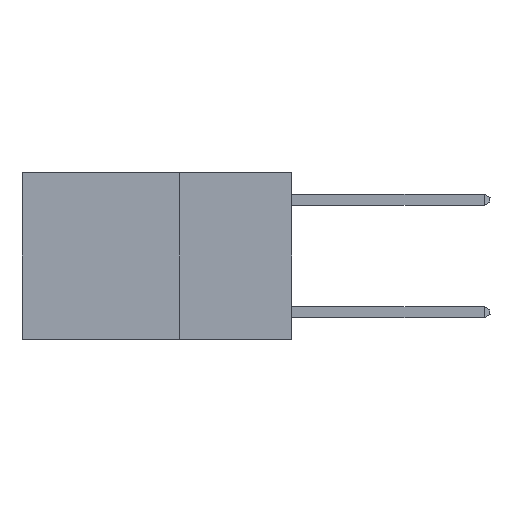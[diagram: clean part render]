
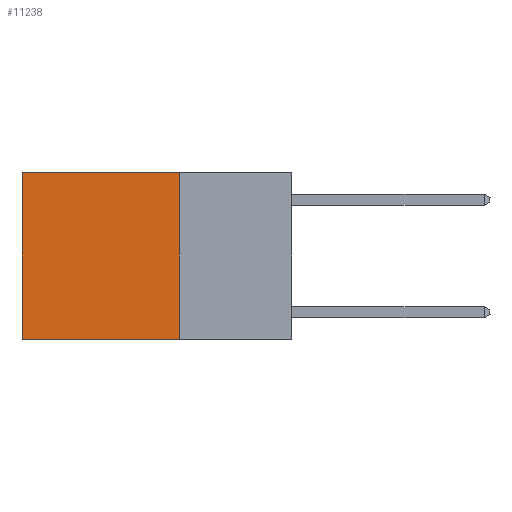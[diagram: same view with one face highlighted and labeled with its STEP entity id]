
A CAD part, left-side view. The second image highlights one B-rep face of the part: STEP entity #11238.
In plain terms, the highlighted planar face has unit normal (-1, 0, 0).
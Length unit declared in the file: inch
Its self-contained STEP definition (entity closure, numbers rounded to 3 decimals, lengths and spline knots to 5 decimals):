
#339 = DIRECTION ( 'NONE',  ( 1., 0., 0. ) ) ;
#448 = VERTEX_POINT ( 'NONE', #9764 ) ;
#543 = ORIENTED_EDGE ( 'NONE', *, *, #3418, .F. ) ;
#803 = CARTESIAN_POINT ( 'NONE',  ( 0.2625, 0.25, 0. ) ) ;
#977 = LINE ( 'NONE', #1709, #9962 ) ;
#1011 = EDGE_CURVE ( 'NONE', #10514, #448, #5418, .T. ) ;
#1025 = LINE ( 'NONE', #6963, #1721 ) ;
#1190 = PLANE ( 'NONE',  #1799 ) ;
#1346 = VECTOR ( 'NONE', #2040, 39.37008 ) ;
#1400 = EDGE_LOOP ( 'NONE', ( #9079, #543, #10496, #2004 ) ) ;
#1709 = CARTESIAN_POINT ( 'NONE',  ( 0.2625, 0.25, -0.37 ) ) ;
#1721 = VECTOR ( 'NONE', #9703, 39.37008 ) ;
#1765 = DIRECTION ( 'NONE',  ( 0., 1., 0. ) ) ;
#1799 = AXIS2_PLACEMENT_3D ( 'NONE', #9866, #339, #7353 ) ;
#1936 = LINE ( 'NONE', #3790, #5682 ) ;
#2004 = ORIENTED_EDGE ( 'NONE', *, *, #7524, .T. ) ;
#2040 = DIRECTION ( 'NONE',  ( 0., 0., -1. ) ) ;
#2879 = DIRECTION ( 'NONE',  ( 0., 1., 0. ) ) ;
#3418 = EDGE_CURVE ( 'NONE', #448, #3503, #977, .T. ) ;
#3503 = VERTEX_POINT ( 'NONE', #10348 ) ;
#3790 = CARTESIAN_POINT ( 'NONE',  ( 0.2625, 0.25, 0. ) ) ;
#3941 = CARTESIAN_POINT ( 'NONE',  ( 0.2625, 0.25, 0. ) ) ;
#5418 = LINE ( 'NONE', #3941, #1346 ) ;
#5682 = VECTOR ( 'NONE', #2879, 39.37008 ) ;
#6334 = VERTEX_POINT ( 'NONE', #6745 ) ;
#6586 = EDGE_CURVE ( 'NONE', #6334, #3503, #1025, .T. ) ;
#6745 = CARTESIAN_POINT ( 'NONE',  ( 0.2625, 0.6, 0. ) ) ;
#6963 = CARTESIAN_POINT ( 'NONE',  ( 0.2625, 0.6, 0. ) ) ;
#7353 = DIRECTION ( 'NONE',  ( 0., 0., -1. ) ) ;
#7524 = EDGE_CURVE ( 'NONE', #10514, #6334, #1936, .T. ) ;
#9008 = FACE_OUTER_BOUND ( 'NONE', #1400, .T. ) ;
#9079 = ORIENTED_EDGE ( 'NONE', *, *, #6586, .T. ) ;
#9703 = DIRECTION ( 'NONE',  ( 0., 0., -1. ) ) ;
#9764 = CARTESIAN_POINT ( 'NONE',  ( 0.2625, 0.25, -0.37 ) ) ;
#9866 = CARTESIAN_POINT ( 'NONE',  ( 0.2625, 0.25, 0. ) ) ;
#9962 = VECTOR ( 'NONE', #1765, 39.37008 ) ;
#10348 = CARTESIAN_POINT ( 'NONE',  ( 0.2625, 0.6, -0.37 ) ) ;
#10496 = ORIENTED_EDGE ( 'NONE', *, *, #1011, .F. ) ;
#10514 = VERTEX_POINT ( 'NONE', #803 ) ;
#11238 = ADVANCED_FACE ( 'NONE', ( #9008 ), #1190, .F. ) ;
